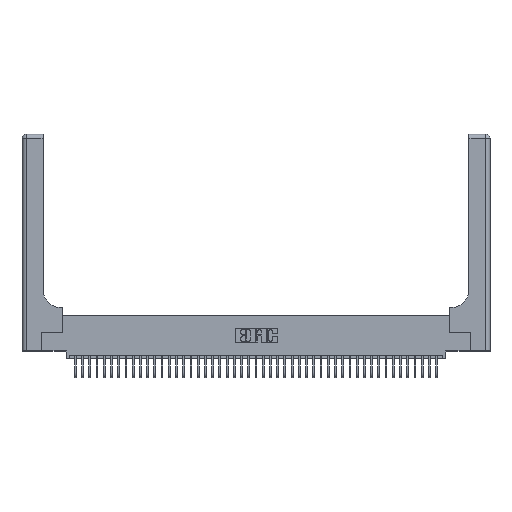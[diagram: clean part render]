
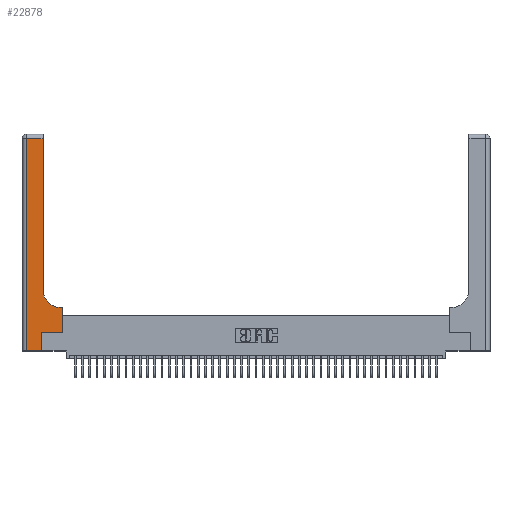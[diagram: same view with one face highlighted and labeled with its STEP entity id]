
A CAD part, top view. The second image highlights one B-rep face of the part: STEP entity #22878.
In plain terms, the highlighted planar face has unit normal (0, 0, 1).
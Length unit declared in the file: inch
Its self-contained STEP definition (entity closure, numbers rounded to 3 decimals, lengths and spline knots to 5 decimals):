
#79 = VECTOR ( 'NONE', #2423, 39.37008 ) ;
#465 = EDGE_LOOP ( 'NONE', ( #27112, #4148, #38186, #30497, #8936, #15054, #30096, #37447, #17658 ) ) ;
#744 = CARTESIAN_POINT ( 'NONE',  ( 0., 2.94, 0.37 ) ) ;
#1622 = VECTOR ( 'NONE', #22944, 39.37008 ) ;
#1968 = AXIS2_PLACEMENT_3D ( 'NONE', #18421, #41281, #21703 ) ;
#2423 = DIRECTION ( 'NONE',  ( 0., 1., 0. ) ) ;
#2857 = DIRECTION ( 'NONE',  ( -1., 0., 0. ) ) ;
#2996 = DIRECTION ( 'NONE',  ( 0., 1., 0. ) ) ;
#3272 = CARTESIAN_POINT ( 'NONE',  ( 0.2915, 0.6, 0.37 ) ) ;
#4116 = VECTOR ( 'NONE', #31774, 39.37008 ) ;
#4140 = DIRECTION ( 'NONE',  ( -1., 0., 0. ) ) ;
#4148 = ORIENTED_EDGE ( 'NONE', *, *, #42065, .T. ) ;
#5924 = DIRECTION ( 'NONE',  ( 0., 1., 0. ) ) ;
#6639 = LINE ( 'NONE', #7093, #14383 ) ;
#7093 = CARTESIAN_POINT ( 'NONE',  ( 0.06, 3., 0.37 ) ) ;
#7586 = VECTOR ( 'NONE', #4140, 39.37008 ) ;
#8657 = CARTESIAN_POINT ( 'NONE',  ( 0.269, 0., 0.37 ) ) ;
#8724 = CARTESIAN_POINT ( 'NONE',  ( 0.269, 0.25, 0.37 ) ) ;
#8936 = ORIENTED_EDGE ( 'NONE', *, *, #14690, .T. ) ;
#9514 = VERTEX_POINT ( 'NONE', #33378 ) ;
#9985 = VECTOR ( 'NONE', #2996, 39.37008 ) ;
#10753 = FACE_OUTER_BOUND ( 'NONE', #465, .T. ) ;
#11474 = LINE ( 'NONE', #42524, #1622 ) ;
#11518 = CARTESIAN_POINT ( 'NONE',  ( 0.5585, 0.25, 0.37 ) ) ;
#11975 = EDGE_CURVE ( 'NONE', #9514, #21494, #6639, .T. ) ;
#12079 = CARTESIAN_POINT ( 'NONE',  ( 0.2915, 0.85, 0.37 ) ) ;
#12876 = LINE ( 'NONE', #8724, #4116 ) ;
#14383 = VECTOR ( 'NONE', #39896, 39.37008 ) ;
#14690 = EDGE_CURVE ( 'NONE', #34064, #36558, #26373, .T. ) ;
#14714 = EDGE_CURVE ( 'NONE', #21974, #41572, #40162, .T. ) ;
#15054 = ORIENTED_EDGE ( 'NONE', *, *, #40599, .T. ) ;
#15618 = VERTEX_POINT ( 'NONE', #39661 ) ;
#15981 = CARTESIAN_POINT ( 'NONE',  ( 0.2915, 2.94, 0.37 ) ) ;
#17064 = EDGE_CURVE ( 'NONE', #41572, #15618, #27152, .T. ) ;
#17288 = AXIS2_PLACEMENT_3D ( 'NONE', #38858, #22556, #2857 ) ;
#17658 = ORIENTED_EDGE ( 'NONE', *, *, #30958, .T. ) ;
#18421 = CARTESIAN_POINT ( 'NONE',  ( 0.5415, 0.85, 0.37 ) ) ;
#18711 = CARTESIAN_POINT ( 'NONE',  ( 0.06, 0., 0.37 ) ) ;
#18729 = LINE ( 'NONE', #32402, #9985 ) ;
#18863 = VERTEX_POINT ( 'NONE', #12079 ) ;
#19683 = DIRECTION ( 'NONE',  ( -1., 0., 0. ) ) ;
#21494 = VERTEX_POINT ( 'NONE', #18711 ) ;
#21703 = DIRECTION ( 'NONE',  ( 1., 0., 0. ) ) ;
#21974 = VERTEX_POINT ( 'NONE', #11518 ) ;
#22556 = DIRECTION ( 'NONE',  ( 0., 0., -1. ) ) ;
#22760 = VECTOR ( 'NONE', #5924, 39.37008 ) ;
#22878 = ADVANCED_FACE ( 'NONE', ( #10753 ), #42147, .F. ) ;
#22944 = DIRECTION ( 'NONE',  ( 1., 0., 0. ) ) ;
#25364 = CARTESIAN_POINT ( 'NONE',  ( 0.269, 0.25, 0.37 ) ) ;
#25429 = CARTESIAN_POINT ( 'NONE',  ( 0.269, 0., 0.37 ) ) ;
#26064 = LINE ( 'NONE', #744, #7586 ) ;
#26373 = LINE ( 'NONE', #25429, #79 ) ;
#26914 = VERTEX_POINT ( 'NONE', #15981 ) ;
#26976 = CARTESIAN_POINT ( 'NONE',  ( 0.5585, 0.6, 0.37 ) ) ;
#27112 = ORIENTED_EDGE ( 'NONE', *, *, #34227, .T. ) ;
#27152 = LINE ( 'NONE', #3272, #34836 ) ;
#27337 = CIRCLE ( 'NONE', #1968, 0.25 ) ;
#30096 = ORIENTED_EDGE ( 'NONE', *, *, #14714, .T. ) ;
#30497 = ORIENTED_EDGE ( 'NONE', *, *, #39141, .T. ) ;
#30958 = EDGE_CURVE ( 'NONE', #15618, #18863, #27337, .T. ) ;
#31774 = DIRECTION ( 'NONE',  ( 1., 0., 0. ) ) ;
#32402 = CARTESIAN_POINT ( 'NONE',  ( 0.2915, 3., 0.37 ) ) ;
#33378 = CARTESIAN_POINT ( 'NONE',  ( 0.06, 2.94, 0.37 ) ) ;
#34064 = VERTEX_POINT ( 'NONE', #8657 ) ;
#34227 = EDGE_CURVE ( 'NONE', #18863, #26914, #18729, .T. ) ;
#34836 = VECTOR ( 'NONE', #19683, 39.37008 ) ;
#36558 = VERTEX_POINT ( 'NONE', #25364 ) ;
#37447 = ORIENTED_EDGE ( 'NONE', *, *, #17064, .T. ) ;
#38186 = ORIENTED_EDGE ( 'NONE', *, *, #11975, .T. ) ;
#38858 = CARTESIAN_POINT ( 'NONE',  ( 0., 3., 0.37 ) ) ;
#39141 = EDGE_CURVE ( 'NONE', #21494, #34064, #11474, .T. ) ;
#39661 = CARTESIAN_POINT ( 'NONE',  ( 0.5415, 0.6, 0.37 ) ) ;
#39896 = DIRECTION ( 'NONE',  ( 0., -1., 0. ) ) ;
#40162 = LINE ( 'NONE', #41869, #22760 ) ;
#40599 = EDGE_CURVE ( 'NONE', #36558, #21974, #12876, .T. ) ;
#41281 = DIRECTION ( 'NONE',  ( 0., 0., -1. ) ) ;
#41572 = VERTEX_POINT ( 'NONE', #26976 ) ;
#41869 = CARTESIAN_POINT ( 'NONE',  ( 0.5585, 0.25, 0.37 ) ) ;
#42065 = EDGE_CURVE ( 'NONE', #26914, #9514, #26064, .T. ) ;
#42147 = PLANE ( 'NONE',  #17288 ) ;
#42524 = CARTESIAN_POINT ( 'NONE',  ( 0., 0., 0.37 ) ) ;
